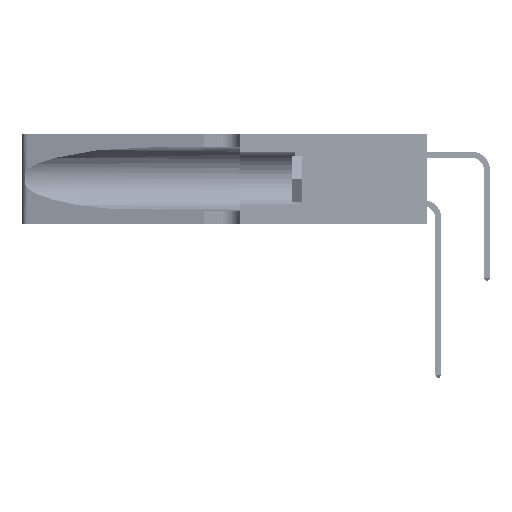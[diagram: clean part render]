
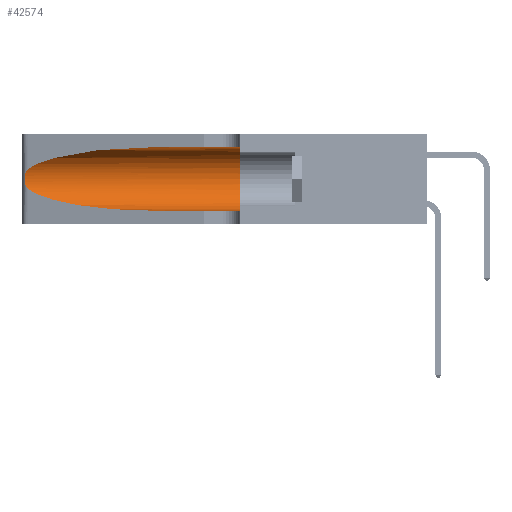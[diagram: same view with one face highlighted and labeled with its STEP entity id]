
A CAD part, left-side view. The second image highlights one B-rep face of the part: STEP entity #42574.
In plain terms, the highlighted cylindrical face has radius 3.308 mm (diameter 6.617 mm), a partial arc.
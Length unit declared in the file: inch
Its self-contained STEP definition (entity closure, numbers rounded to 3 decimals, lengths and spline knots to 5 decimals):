
#1534 = AXIS2_PLACEMENT_3D ( 'NONE', #27421, #35351, #43327 ) ;
#2254 = CARTESIAN_POINT ( 'NONE',  ( 0.25555, 1.22994, 0.2215 ) ) ;
#2426 = CARTESIAN_POINT ( 'NONE',  ( 0.26075, 1.23896, 0.19203 ) ) ;
#3182 = VERTEX_POINT ( 'NONE', #32654 ) ;
#3595 = ORIENTED_EDGE ( 'NONE', *, *, #19175, .T. ) ;
#4504 = CIRCLE ( 'NONE', #19941, 0.13025 ) ;
#6535 = CARTESIAN_POINT ( 'NONE',  ( 0.26017, 1.23833, 0.17102 ) ) ;
#6545 = VERTEX_POINT ( 'NONE', #11840 ) ;
#7364 = CARTESIAN_POINT ( 'NONE',  ( 0.18966, 0.96281, 0.31525 ) ) ;
#8508 = EDGE_CURVE ( 'NONE', #36449, #21873, #25167, .T. ) ;
#9774 = VERTEX_POINT ( 'NONE', #37004 ) ;
#9913 = ORIENTED_EDGE ( 'NONE', *, *, #12080, .F. ) ;
#10576 = CARTESIAN_POINT ( 'NONE',  ( 0.25789, 1.23486, 0.15765 ) ) ;
#11840 = CARTESIAN_POINT ( 'NONE',  ( 0.25487, 1.22718, 0.14631 ) ) ;
#12080 = EDGE_CURVE ( 'NONE', #21873, #31951, #4504, .T. ) ;
#13077 = ORIENTED_EDGE ( 'NONE', *, *, #24473, .T. ) ;
#13512 = CARTESIAN_POINT ( 'NONE',  ( 0.1305, 0.35, 0.185 ) ) ;
#14654 = CARTESIAN_POINT ( 'NONE',  ( 0.25555, 1.22993, 0.14849 ) ) ;
#15491 = CARTESIAN_POINT ( 'NONE',  ( 0.25487, 1.22718, 0.22369 ) ) ;
#15715 = CARTESIAN_POINT ( 'NONE',  ( 0.1305, 1.61858, 0.05475 ) ) ;
#17581 = DIRECTION ( 'NONE',  ( 0., 0., 1. ) ) ;
#18228 = CARTESIAN_POINT ( 'NONE',  ( 0.1305, 0.35, 0.05475 ) ) ;
#19010 = CARTESIAN_POINT ( 'NONE',  ( 0.1305, 0.72297, 0.31525 ) ) ;
#19175 = EDGE_CURVE ( 'NONE', #3182, #6545, #48521, .T. ) ;
#19781 = DIRECTION ( 'NONE',  ( 0., -1., 0. ) ) ;
#19835 = CARTESIAN_POINT ( 'NONE',  ( 0.25487, 1.22718, 0.14631 ) ) ;
#19941 = AXIS2_PLACEMENT_3D ( 'NONE', #13512, #41419, #17581 ) ;
#21873 = VERTEX_POINT ( 'NONE', #43864 ) ;
#21974 = VECTOR ( 'NONE', #19781, 39.37008 ) ;
#22603 = CARTESIAN_POINT ( 'NONE',  ( 0.25787, 1.23484, 0.2124 ) ) ;
#23130 = CYLINDRICAL_SURFACE ( 'NONE', #1534, 0.13025 ) ;
#23261 = CARTESIAN_POINT ( 'NONE',  ( 0.1305, 0.72297, 0.31525 ) ) ;
#23881 = CARTESIAN_POINT ( 'NONE',  ( 0.18966, 0.96281, 0.05475 ) ) ;
#24473 = EDGE_CURVE ( 'NONE', #36449, #3182, #30100, .T. ) ;
#25167 = LINE ( 'NONE', #25193, #33223 ) ;
#25193 = CARTESIAN_POINT ( 'NONE',  ( 0.1305, 1.61858, 0.31525 ) ) ;
#26625 = CARTESIAN_POINT ( 'NONE',  ( 0.26018, 1.23835, 0.19895 ) ) ;
#27421 = CARTESIAN_POINT ( 'NONE',  ( 0.1305, 1.61858, 0.185 ) ) ;
#27580 = ORIENTED_EDGE ( 'NONE', *, *, #45937, .T. ) ;
#30100 =( BOUNDED_CURVE ( )  B_SPLINE_CURVE ( 3, ( #23261, #7364, #39377, #15491 ),
 .UNSPECIFIED., .F., .T. ) 
 B_SPLINE_CURVE_WITH_KNOTS ( ( 4, 4 ),
 ( 1.5708, 2.84003 ),
 .UNSPECIFIED. ) 
 CURVE ( )  GEOMETRIC_REPRESENTATION_ITEM ( )  RATIONAL_B_SPLINE_CURVE ( ( 1., 0.87, 0.87, 1. ) ) 
 REPRESENTATION_ITEM ( '' )  );
#30604 = CARTESIAN_POINT ( 'NONE',  ( 0.26075, 1.23896, 0.178 ) ) ;
#31313 = ORIENTED_EDGE ( 'NONE', *, *, #8508, .F. ) ;
#31951 = VERTEX_POINT ( 'NONE', #18228 ) ;
#32654 = CARTESIAN_POINT ( 'NONE',  ( 0.25487, 1.22718, 0.22369 ) ) ;
#32894 = EDGE_LOOP ( 'NONE', ( #13077, #3595, #47402, #27580, #9913, #31313 ) ) ;
#33223 = VECTOR ( 'NONE', #49081, 39.37008 ) ;
#34569 = CARTESIAN_POINT ( 'NONE',  ( 0.25856, 1.23593, 0.16098 ) ) ;
#35351 = DIRECTION ( 'NONE',  ( 0., -1., 0. ) ) ;
#36268 = LINE ( 'NONE', #15715, #21974 ) ;
#36449 = VERTEX_POINT ( 'NONE', #19010 ) ;
#37004 = CARTESIAN_POINT ( 'NONE',  ( 0.1305, 0.72297, 0.05475 ) ) ;
#38534 = CARTESIAN_POINT ( 'NONE',  ( 0.25639, 1.23186, 0.15144 ) ) ;
#39188 = EDGE_CURVE ( 'NONE', #6545, #9774, #50096, .T. ) ;
#39377 = CARTESIAN_POINT ( 'NONE',  ( 0.2373, 1.15595, 0.28018 ) ) ;
#41419 = DIRECTION ( 'NONE',  ( 0., 1., 0. ) ) ;
#42546 = CARTESIAN_POINT ( 'NONE',  ( 0.25487, 1.22718, 0.14631 ) ) ;
#42574 = ADVANCED_FACE ( 'NONE', ( #44240 ), #23130, .F. ) ;
#43327 = DIRECTION ( 'NONE',  ( 0., 0., -1. ) ) ;
#43640 = CARTESIAN_POINT ( 'NONE',  ( 0.2373, 1.15595, 0.08982 ) ) ;
#43864 = CARTESIAN_POINT ( 'NONE',  ( 0.1305, 0.35, 0.31525 ) ) ;
#44240 = FACE_OUTER_BOUND ( 'NONE', #32894, .T. ) ;
#45937 = EDGE_CURVE ( 'NONE', #9774, #31951, #36268, .T. ) ;
#46379 = CARTESIAN_POINT ( 'NONE',  ( 0.25639, 1.23184, 0.21858 ) ) ;
#47402 = ORIENTED_EDGE ( 'NONE', *, *, #39188, .T. ) ;
#48521 = B_SPLINE_CURVE_WITH_KNOTS ( 'NONE', 3,
 ( #50158, #2254, #46379, #22603, #50336, #26625, #2426, #30604, #6535, #34569, #10576, #38534, #14654, #42546 ),
 .UNSPECIFIED., .F., .F.,
 ( 4, 2, 2, 2, 2, 2, 4 ),
 ( 0., 0.00027, 0.00053, 0.00107, 0.0016, 0.00187, 0.00214 ),
 .UNSPECIFIED. ) ;
#49081 = DIRECTION ( 'NONE',  ( 0., -1., 0. ) ) ;
#50096 =( BOUNDED_CURVE ( )  B_SPLINE_CURVE ( 3, ( #19835, #43640, #23881, #51593 ),
 .UNSPECIFIED., .F., .F. ) 
 B_SPLINE_CURVE_WITH_KNOTS ( ( 4, 4 ),
 ( 3.44316, 4.71239 ),
 .UNSPECIFIED. ) 
 CURVE ( )  GEOMETRIC_REPRESENTATION_ITEM ( )  RATIONAL_B_SPLINE_CURVE ( ( 1., 0.87, 0.87, 1. ) ) 
 REPRESENTATION_ITEM ( '' )  );
#50158 = CARTESIAN_POINT ( 'NONE',  ( 0.25487, 1.22718, 0.22369 ) ) ;
#50336 = CARTESIAN_POINT ( 'NONE',  ( 0.25854, 1.2359, 0.20912 ) ) ;
#51593 = CARTESIAN_POINT ( 'NONE',  ( 0.1305, 0.72297, 0.05475 ) ) ;
